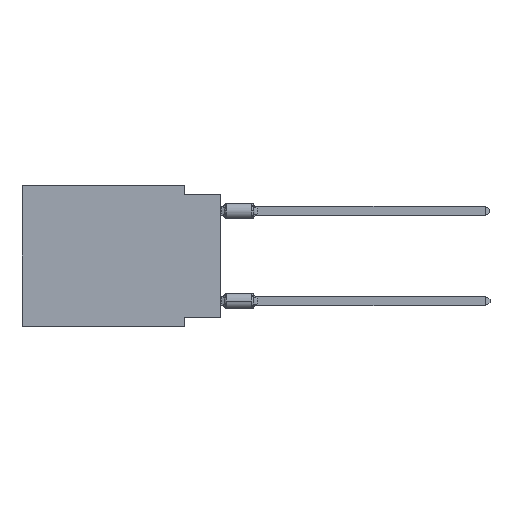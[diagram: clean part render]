
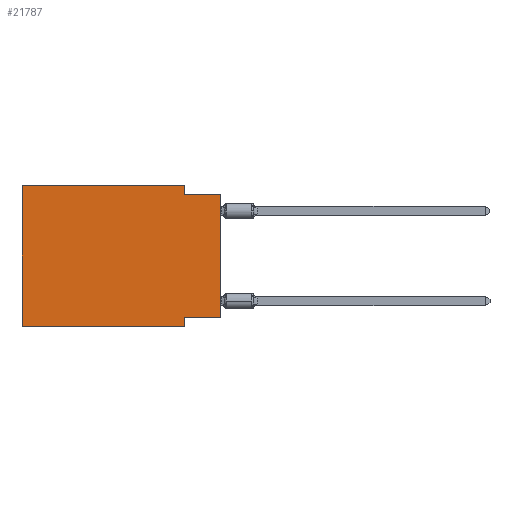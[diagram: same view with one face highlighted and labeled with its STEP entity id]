
A CAD part, left-side view. The second image highlights one B-rep face of the part: STEP entity #21787.
In plain terms, the highlighted planar face has unit normal (-1, 0, 0).
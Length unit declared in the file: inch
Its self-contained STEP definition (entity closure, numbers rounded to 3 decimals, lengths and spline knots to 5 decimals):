
#654 = VERTEX_POINT ( 'NONE', #3733 ) ;
#732 = VECTOR ( 'NONE', #23173, 39.37008 ) ;
#844 = EDGE_LOOP ( 'NONE', ( #8898, #12512, #20464, #4826, #25994, #18812, #20090, #23279 ) ) ;
#888 = CARTESIAN_POINT ( 'NONE',  ( 0., 0.55, 0. ) ) ;
#941 = CARTESIAN_POINT ( 'NONE',  ( 0., 0.1, -0.025 ) ) ;
#1492 = CARTESIAN_POINT ( 'NONE',  ( 0., 0.55, -0.39 ) ) ;
#1700 = DIRECTION ( 'NONE',  ( 0., -1., 0. ) ) ;
#2523 = DIRECTION ( 'NONE',  ( 0., 0., -1. ) ) ;
#3115 = CARTESIAN_POINT ( 'NONE',  ( 0., 0.1, -0.365 ) ) ;
#3370 = PLANE ( 'NONE',  #25479 ) ;
#3733 = CARTESIAN_POINT ( 'NONE',  ( 0., 0.1, 0. ) ) ;
#4164 = EDGE_CURVE ( 'NONE', #19205, #14749, #12138, .T. ) ;
#4819 = EDGE_CURVE ( 'NONE', #11081, #14749, #19298, .T. ) ;
#4826 = ORIENTED_EDGE ( 'NONE', *, *, #26277, .F. ) ;
#5032 = VECTOR ( 'NONE', #2523, 39.37008 ) ;
#5550 = FACE_OUTER_BOUND ( 'NONE', #844, .T. ) ;
#5690 = CARTESIAN_POINT ( 'NONE',  ( 0., 0.55, 0. ) ) ;
#6245 = VERTEX_POINT ( 'NONE', #14077 ) ;
#6251 = DIRECTION ( 'NONE',  ( 0., -1., 0. ) ) ;
#7052 = VECTOR ( 'NONE', #1700, 39.37008 ) ;
#7293 = VECTOR ( 'NONE', #21966, 39.37008 ) ;
#8279 = EDGE_CURVE ( 'NONE', #17925, #6245, #22442, .T. ) ;
#8390 = CARTESIAN_POINT ( 'NONE',  ( 0., 0.55, 0. ) ) ;
#8803 = EDGE_CURVE ( 'NONE', #25497, #6245, #17047, .T. ) ;
#8898 = ORIENTED_EDGE ( 'NONE', *, *, #8279, .T. ) ;
#9082 = CARTESIAN_POINT ( 'NONE',  ( 0., 0.1, -0.39 ) ) ;
#9671 = VECTOR ( 'NONE', #26518, 39.37008 ) ;
#9916 = CARTESIAN_POINT ( 'NONE',  ( 0., 0.1, 0. ) ) ;
#9994 = CARTESIAN_POINT ( 'NONE',  ( 0., 0.55, 0. ) ) ;
#10583 = EDGE_CURVE ( 'NONE', #17925, #11081, #11755, .T. ) ;
#11081 = VERTEX_POINT ( 'NONE', #3115 ) ;
#11755 = LINE ( 'NONE', #20050, #7293 ) ;
#11982 = LINE ( 'NONE', #8390, #7052 ) ;
#12058 = LINE ( 'NONE', #9994, #13644 ) ;
#12138 = LINE ( 'NONE', #14184, #26101 ) ;
#12512 = ORIENTED_EDGE ( 'NONE', *, *, #8803, .F. ) ;
#13644 = VECTOR ( 'NONE', #22652, 39.37008 ) ;
#13874 = CARTESIAN_POINT ( 'NONE',  ( 0., 0., -0.365 ) ) ;
#14077 = CARTESIAN_POINT ( 'NONE',  ( 0., 0., -0.025 ) ) ;
#14148 = DIRECTION ( 'NONE',  ( 0., 0., 1. ) ) ;
#14184 = CARTESIAN_POINT ( 'NONE',  ( 0., 0.55, -0.39 ) ) ;
#14279 = LINE ( 'NONE', #9916, #9671 ) ;
#14749 = VERTEX_POINT ( 'NONE', #9082 ) ;
#15655 = DIRECTION ( 'NONE',  ( 1., 0., 0. ) ) ;
#16191 = CARTESIAN_POINT ( 'NONE',  ( 0., 0., 0. ) ) ;
#16523 = VECTOR ( 'NONE', #14148, 39.37008 ) ;
#16919 = CARTESIAN_POINT ( 'NONE',  ( 0., 0., -0.025 ) ) ;
#17047 = LINE ( 'NONE', #16919, #732 ) ;
#17925 = VERTEX_POINT ( 'NONE', #13874 ) ;
#17950 = VERTEX_POINT ( 'NONE', #5690 ) ;
#18812 = ORIENTED_EDGE ( 'NONE', *, *, #4164, .T. ) ;
#18906 = EDGE_CURVE ( 'NONE', #19205, #17950, #12058, .T. ) ;
#19205 = VERTEX_POINT ( 'NONE', #1492 ) ;
#19298 = LINE ( 'NONE', #21197, #5032 ) ;
#20050 = CARTESIAN_POINT ( 'NONE',  ( 0., 0., -0.365 ) ) ;
#20090 = ORIENTED_EDGE ( 'NONE', *, *, #4819, .F. ) ;
#20464 = ORIENTED_EDGE ( 'NONE', *, *, #26330, .F. ) ;
#21197 = CARTESIAN_POINT ( 'NONE',  ( 0., 0.1, -0.39 ) ) ;
#21787 = ADVANCED_FACE ( 'NONE', ( #5550 ), #3370, .F. ) ;
#21966 = DIRECTION ( 'NONE',  ( 0., 1., 0. ) ) ;
#22442 = LINE ( 'NONE', #16191, #16523 ) ;
#22652 = DIRECTION ( 'NONE',  ( 0., 0., 1. ) ) ;
#23173 = DIRECTION ( 'NONE',  ( 0., -1., 0. ) ) ;
#23279 = ORIENTED_EDGE ( 'NONE', *, *, #10583, .F. ) ;
#25479 = AXIS2_PLACEMENT_3D ( 'NONE', #888, #15655, #26115 ) ;
#25497 = VERTEX_POINT ( 'NONE', #941 ) ;
#25994 = ORIENTED_EDGE ( 'NONE', *, *, #18906, .F. ) ;
#26101 = VECTOR ( 'NONE', #6251, 39.37008 ) ;
#26115 = DIRECTION ( 'NONE',  ( 0., 0., -1. ) ) ;
#26277 = EDGE_CURVE ( 'NONE', #17950, #654, #11982, .T. ) ;
#26330 = EDGE_CURVE ( 'NONE', #654, #25497, #14279, .T. ) ;
#26518 = DIRECTION ( 'NONE',  ( 0., 0., -1. ) ) ;
